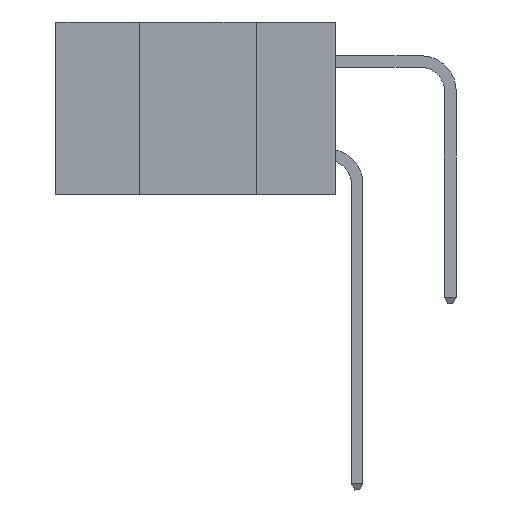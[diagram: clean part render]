
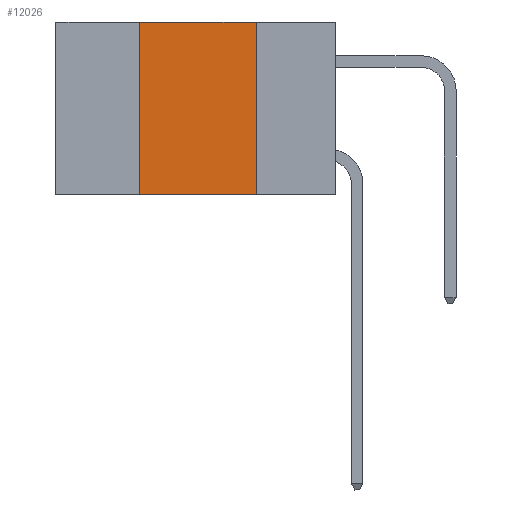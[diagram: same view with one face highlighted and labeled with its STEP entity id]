
A CAD part, left-side view. The second image highlights one B-rep face of the part: STEP entity #12026.
In plain terms, the highlighted planar face has unit normal (-1, 0, 0).
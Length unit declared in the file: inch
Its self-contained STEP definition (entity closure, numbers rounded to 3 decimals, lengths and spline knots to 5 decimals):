
#921 = DIRECTION ( 'NONE',  ( 1., 0., 0. ) ) ;
#1151 = AXIS2_PLACEMENT_3D ( 'NONE', #17753, #921, #14225 ) ;
#1705 = VERTEX_POINT ( 'NONE', #20043 ) ;
#2215 = EDGE_CURVE ( 'NONE', #1705, #4026, #4817, .T. ) ;
#2865 = ORIENTED_EDGE ( 'NONE', *, *, #19190, .F. ) ;
#4026 = VERTEX_POINT ( 'NONE', #4672 ) ;
#4672 = CARTESIAN_POINT ( 'NONE',  ( 0., 0.42, 0. ) ) ;
#4679 = CARTESIAN_POINT ( 'NONE',  ( 0., 0.17, -0.37 ) ) ;
#4680 = VECTOR ( 'NONE', #15839, 39.37008 ) ;
#4817 = LINE ( 'NONE', #20418, #14185 ) ;
#6032 = CARTESIAN_POINT ( 'NONE',  ( 0., 0.6, -0.37 ) ) ;
#9385 = LINE ( 'NONE', #10946, #23321 ) ;
#9817 = LINE ( 'NONE', #19460, #4680 ) ;
#10448 = EDGE_CURVE ( 'NONE', #1705, #18224, #13317, .T. ) ;
#10946 = CARTESIAN_POINT ( 'NONE',  ( 0., 0.17, 0. ) ) ;
#12026 = ADVANCED_FACE ( 'NONE', ( #20327 ), #23294, .F. ) ;
#13005 = ORIENTED_EDGE ( 'NONE', *, *, #2215, .F. ) ;
#13317 = LINE ( 'NONE', #6032, #22389 ) ;
#13442 = DIRECTION ( 'NONE',  ( 0., 0., 1. ) ) ;
#13495 = EDGE_LOOP ( 'NONE', ( #22054, #2865, #13005, #17771 ) ) ;
#14091 = VERTEX_POINT ( 'NONE', #24231 ) ;
#14185 = VECTOR ( 'NONE', #13442, 39.37008 ) ;
#14225 = DIRECTION ( 'NONE',  ( 0., 0., -1. ) ) ;
#15768 = EDGE_CURVE ( 'NONE', #14091, #18224, #9385, .T. ) ;
#15839 = DIRECTION ( 'NONE',  ( 0., -1., 0. ) ) ;
#17753 = CARTESIAN_POINT ( 'NONE',  ( 0., 0.6, 0. ) ) ;
#17771 = ORIENTED_EDGE ( 'NONE', *, *, #10448, .T. ) ;
#18224 = VERTEX_POINT ( 'NONE', #4679 ) ;
#18870 = DIRECTION ( 'NONE',  ( 0., -1., 0. ) ) ;
#19190 = EDGE_CURVE ( 'NONE', #4026, #14091, #9817, .T. ) ;
#19460 = CARTESIAN_POINT ( 'NONE',  ( 0., 0.6, 0. ) ) ;
#19965 = DIRECTION ( 'NONE',  ( 0., 0., -1. ) ) ;
#20043 = CARTESIAN_POINT ( 'NONE',  ( 0., 0.42, -0.37 ) ) ;
#20327 = FACE_OUTER_BOUND ( 'NONE', #13495, .T. ) ;
#20418 = CARTESIAN_POINT ( 'NONE',  ( 0., 0.42, 0. ) ) ;
#22054 = ORIENTED_EDGE ( 'NONE', *, *, #15768, .F. ) ;
#22389 = VECTOR ( 'NONE', #18870, 39.37008 ) ;
#23294 = PLANE ( 'NONE',  #1151 ) ;
#23321 = VECTOR ( 'NONE', #19965, 39.37008 ) ;
#24231 = CARTESIAN_POINT ( 'NONE',  ( 0., 0.17, 0. ) ) ;
